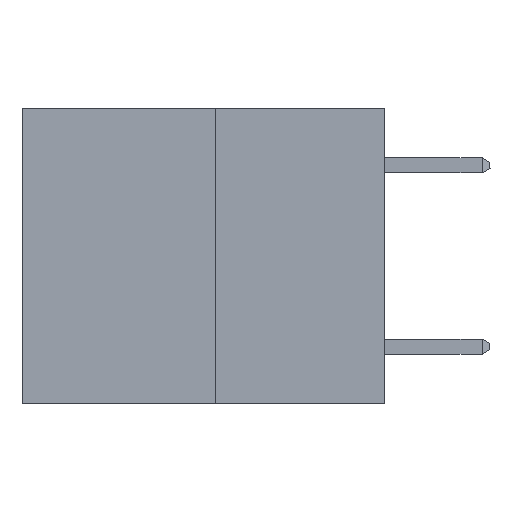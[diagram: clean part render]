
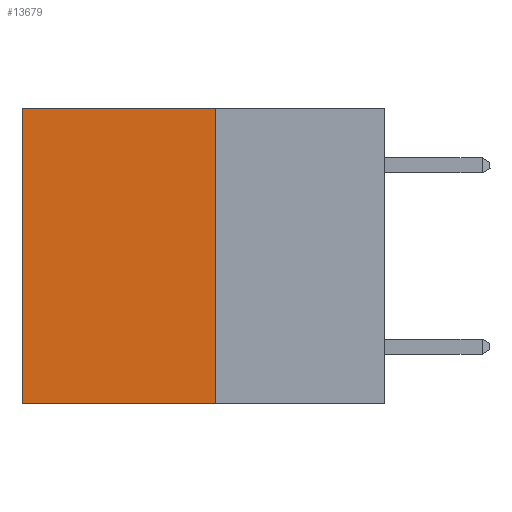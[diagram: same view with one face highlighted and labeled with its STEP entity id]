
A CAD part, left-side view. The second image highlights one B-rep face of the part: STEP entity #13679.
In plain terms, the highlighted planar face has unit normal (-1, 0, 0).
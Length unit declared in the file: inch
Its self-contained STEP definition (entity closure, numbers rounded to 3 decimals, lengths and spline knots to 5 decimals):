
#1601 = EDGE_CURVE ( 'NONE', #11816, #11862, #5518, .T. ) ;
#3298 = ORIENTED_EDGE ( 'NONE', *, *, #6584, .T. ) ;
#3795 = CARTESIAN_POINT ( 'NONE',  ( 0.3165, 0.28, -0.49 ) ) ;
#3947 = EDGE_CURVE ( 'NONE', #7255, #11862, #13163, .T. ) ;
#5053 = DIRECTION ( 'NONE',  ( 0., 1., 0. ) ) ;
#5191 = ORIENTED_EDGE ( 'NONE', *, *, #1601, .F. ) ;
#5518 = LINE ( 'NONE', #15675, #7178 ) ;
#6417 = VECTOR ( 'NONE', #13178, 39.37008 ) ;
#6584 = EDGE_CURVE ( 'NONE', #6587, #7255, #15554, .T. ) ;
#6587 = VERTEX_POINT ( 'NONE', #16260 ) ;
#7178 = VECTOR ( 'NONE', #5053, 39.37008 ) ;
#7255 = VERTEX_POINT ( 'NONE', #9970 ) ;
#7362 = DIRECTION ( 'NONE',  ( 0., 0., -1. ) ) ;
#9159 = CARTESIAN_POINT ( 'NONE',  ( 0.3165, 0.28, 0. ) ) ;
#9756 = FACE_OUTER_BOUND ( 'NONE', #20438, .T. ) ;
#9970 = CARTESIAN_POINT ( 'NONE',  ( 0.3165, 0.6, 0. ) ) ;
#10851 = DIRECTION ( 'NONE',  ( 1., 0., 0. ) ) ;
#11816 = VERTEX_POINT ( 'NONE', #17797 ) ;
#11862 = VERTEX_POINT ( 'NONE', #17691 ) ;
#11920 = CARTESIAN_POINT ( 'NONE',  ( 0.3165, 0.6, -0.49 ) ) ;
#12744 = VECTOR ( 'NONE', #14455, 39.37008 ) ;
#12833 = PLANE ( 'NONE',  #18528 ) ;
#13163 = LINE ( 'NONE', #11920, #22625 ) ;
#13178 = DIRECTION ( 'NONE',  ( 0., 0., -1. ) ) ;
#13225 = ORIENTED_EDGE ( 'NONE', *, *, #3947, .T. ) ;
#13679 = ADVANCED_FACE ( 'NONE', ( #9756 ), #12833, .F. ) ;
#14455 = DIRECTION ( 'NONE',  ( 0., 1., 0. ) ) ;
#15554 = LINE ( 'NONE', #9159, #12744 ) ;
#15675 = CARTESIAN_POINT ( 'NONE',  ( 0.3165, 0.28, -0.49 ) ) ;
#16260 = CARTESIAN_POINT ( 'NONE',  ( 0.3165, 0.28, 0. ) ) ;
#16403 = LINE ( 'NONE', #22065, #6417 ) ;
#17691 = CARTESIAN_POINT ( 'NONE',  ( 0.3165, 0.6, -0.49 ) ) ;
#17797 = CARTESIAN_POINT ( 'NONE',  ( 0.3165, 0.28, -0.49 ) ) ;
#17836 = EDGE_CURVE ( 'NONE', #6587, #11816, #16403, .T. ) ;
#18528 = AXIS2_PLACEMENT_3D ( 'NONE', #3795, #10851, #7362 ) ;
#20438 = EDGE_LOOP ( 'NONE', ( #13225, #5191, #21092, #3298 ) ) ;
#21092 = ORIENTED_EDGE ( 'NONE', *, *, #17836, .F. ) ;
#22065 = CARTESIAN_POINT ( 'NONE',  ( 0.3165, 0.28, -0.49 ) ) ;
#22625 = VECTOR ( 'NONE', #22939, 39.37008 ) ;
#22939 = DIRECTION ( 'NONE',  ( 0., 0., -1. ) ) ;
